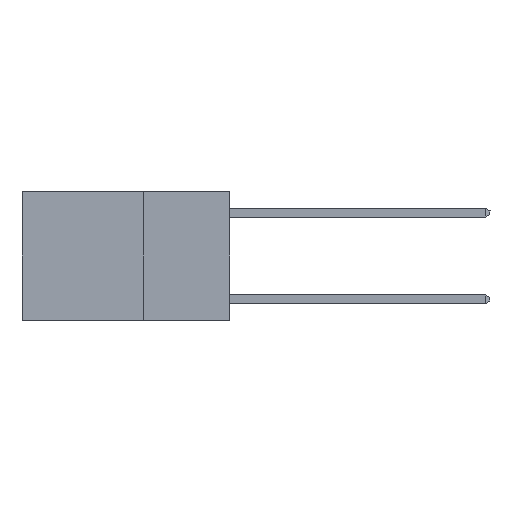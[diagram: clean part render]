
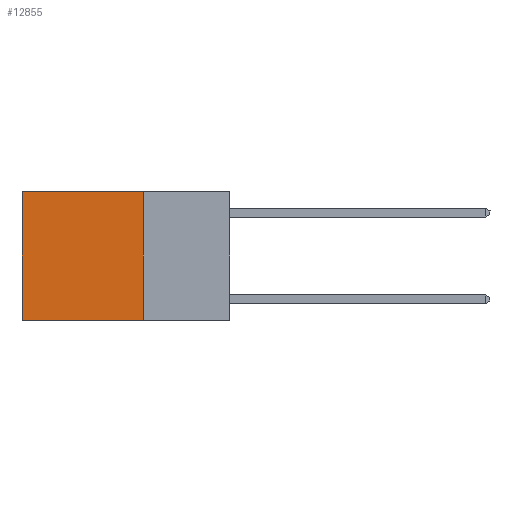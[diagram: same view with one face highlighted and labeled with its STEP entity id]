
A CAD part, left-side view. The second image highlights one B-rep face of the part: STEP entity #12855.
In plain terms, the highlighted planar face has unit normal (-1, 0, 0).
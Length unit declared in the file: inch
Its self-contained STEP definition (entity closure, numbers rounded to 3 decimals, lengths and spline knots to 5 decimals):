
#208 = VECTOR ( 'NONE', #5594, 39.37008 ) ;
#637 = DIRECTION ( 'NONE',  ( 0., 0., -1. ) ) ;
#1561 = ORIENTED_EDGE ( 'NONE', *, *, #14444, .T. ) ;
#2577 = AXIS2_PLACEMENT_3D ( 'NONE', #16200, #21664, #637 ) ;
#3170 = VERTEX_POINT ( 'NONE', #14276 ) ;
#4019 = PLANE ( 'NONE',  #2577 ) ;
#4034 = CARTESIAN_POINT ( 'NONE',  ( 0.2625, 0.25, -0.37 ) ) ;
#5155 = CARTESIAN_POINT ( 'NONE',  ( 0.2625, 0.6, 0. ) ) ;
#5594 = DIRECTION ( 'NONE',  ( 0., 0., -1. ) ) ;
#5880 = ORIENTED_EDGE ( 'NONE', *, *, #19719, .F. ) ;
#5910 = CARTESIAN_POINT ( 'NONE',  ( 0.2625, 0.6, 0. ) ) ;
#6065 = CARTESIAN_POINT ( 'NONE',  ( 0.2625, 0.25, -0.37 ) ) ;
#6282 = LINE ( 'NONE', #6065, #9222 ) ;
#6863 = DIRECTION ( 'NONE',  ( 0., 1., 0. ) ) ;
#9149 = FACE_OUTER_BOUND ( 'NONE', #20982, .T. ) ;
#9222 = VECTOR ( 'NONE', #18256, 39.37008 ) ;
#9522 = VECTOR ( 'NONE', #6863, 39.37008 ) ;
#11067 = VERTEX_POINT ( 'NONE', #11501 ) ;
#11501 = CARTESIAN_POINT ( 'NONE',  ( 0.2625, 0.6, -0.37 ) ) ;
#11903 = DIRECTION ( 'NONE',  ( 0., 0., -1. ) ) ;
#12855 = ADVANCED_FACE ( 'NONE', ( #9149 ), #4019, .F. ) ;
#14276 = CARTESIAN_POINT ( 'NONE',  ( 0.2625, 0.25, 0. ) ) ;
#14444 = EDGE_CURVE ( 'NONE', #3170, #15223, #20438, .T. ) ;
#15223 = VERTEX_POINT ( 'NONE', #5910 ) ;
#15450 = LINE ( 'NONE', #17389, #17244 ) ;
#15783 = EDGE_CURVE ( 'NONE', #3170, #15858, #15450, .T. ) ;
#15842 = LINE ( 'NONE', #5155, #208 ) ;
#15858 = VERTEX_POINT ( 'NONE', #4034 ) ;
#16200 = CARTESIAN_POINT ( 'NONE',  ( 0.2625, 0.25, 0. ) ) ;
#16855 = EDGE_CURVE ( 'NONE', #15223, #11067, #15842, .T. ) ;
#17244 = VECTOR ( 'NONE', #11903, 39.37008 ) ;
#17389 = CARTESIAN_POINT ( 'NONE',  ( 0.2625, 0.25, 0. ) ) ;
#18256 = DIRECTION ( 'NONE',  ( 0., 1., 0. ) ) ;
#18932 = ORIENTED_EDGE ( 'NONE', *, *, #16855, .T. ) ;
#19719 = EDGE_CURVE ( 'NONE', #15858, #11067, #6282, .T. ) ;
#20438 = LINE ( 'NONE', #20655, #9522 ) ;
#20655 = CARTESIAN_POINT ( 'NONE',  ( 0.2625, 0.25, 0. ) ) ;
#20982 = EDGE_LOOP ( 'NONE', ( #18932, #5880, #22033, #1561 ) ) ;
#21664 = DIRECTION ( 'NONE',  ( 1., 0., 0. ) ) ;
#22033 = ORIENTED_EDGE ( 'NONE', *, *, #15783, .F. ) ;
